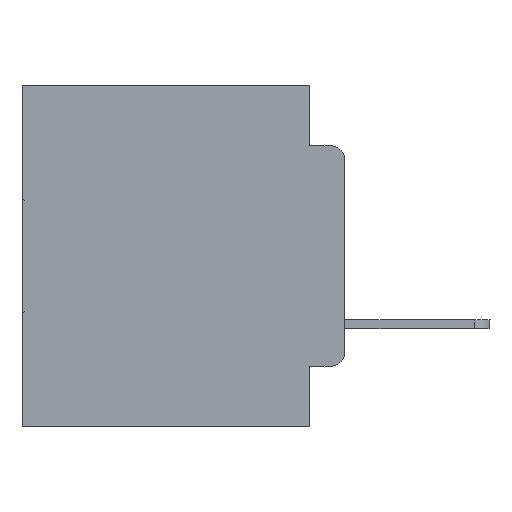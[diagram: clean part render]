
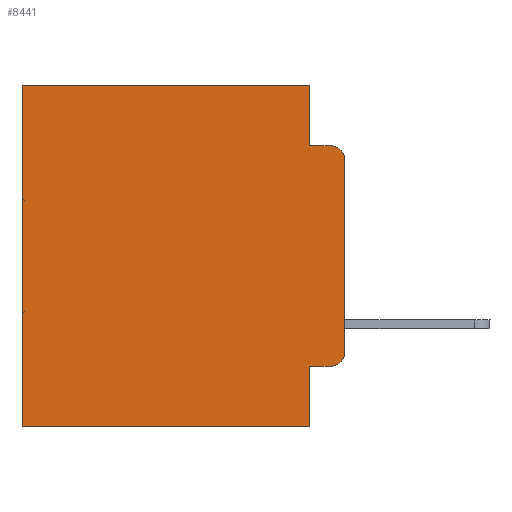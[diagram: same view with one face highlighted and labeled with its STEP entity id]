
A CAD part, left-side view. The second image highlights one B-rep face of the part: STEP entity #8441.
In plain terms, the highlighted planar face has unit normal (-1, 0, 0).
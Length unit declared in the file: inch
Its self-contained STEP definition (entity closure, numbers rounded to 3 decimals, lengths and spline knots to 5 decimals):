
#83 = DIRECTION ( 'NONE',  ( 0., 0., -1. ) ) ;
#173 = VERTEX_POINT ( 'NONE', #23700 ) ;
#396 = EDGE_CURVE ( 'NONE', #19547, #23823, #25147, .T. ) ;
#588 = EDGE_LOOP ( 'NONE', ( #3178, #11510, #20989, #927, #28662, #27290, #29901, #21959, #3169, #2044 ) ) ;
#727 = VECTOR ( 'NONE', #8855, 39.37008 ) ;
#927 = ORIENTED_EDGE ( 'NONE', *, *, #28316, .F. ) ;
#1236 = DIRECTION ( 'NONE',  ( 1., 0., 0. ) ) ;
#1614 = CARTESIAN_POINT ( 'NONE',  ( 0.298, 0.473, -0.5 ) ) ;
#1920 = CARTESIAN_POINT ( 'NONE',  ( 0.298, 0.051, -0.0885 ) ) ;
#2044 = ORIENTED_EDGE ( 'NONE', *, *, #396, .T. ) ;
#2188 = CARTESIAN_POINT ( 'NONE',  ( 0.298, 0.051, 0. ) ) ;
#2474 = CARTESIAN_POINT ( 'NONE',  ( 0.298, 0.473, 0. ) ) ;
#2804 = DIRECTION ( 'NONE',  ( 0., 0., -1. ) ) ;
#3169 = ORIENTED_EDGE ( 'NONE', *, *, #11675, .T. ) ;
#3178 = ORIENTED_EDGE ( 'NONE', *, *, #8367, .F. ) ;
#3919 = LINE ( 'NONE', #23243, #4625 ) ;
#4054 = VERTEX_POINT ( 'NONE', #20038 ) ;
#4377 = CARTESIAN_POINT ( 'NONE',  ( 0.298, 0.051, -0.4115 ) ) ;
#4625 = VECTOR ( 'NONE', #15830, 39.37008 ) ;
#4672 = LINE ( 'NONE', #16582, #15466 ) ;
#4869 = EDGE_CURVE ( 'NONE', #14816, #173, #23444, .T. ) ;
#5251 = VECTOR ( 'NONE', #28047, 39.37008 ) ;
#5938 = DIRECTION ( 'NONE',  ( -1., 0., 0. ) ) ;
#7000 = CARTESIAN_POINT ( 'NONE',  ( 0.298, 0.473, 0. ) ) ;
#7826 = VERTEX_POINT ( 'NONE', #1614 ) ;
#7828 = VERTEX_POINT ( 'NONE', #1920 ) ;
#8042 = VERTEX_POINT ( 'NONE', #24629 ) ;
#8151 = EDGE_CURVE ( 'NONE', #8042, #12135, #10025, .T. ) ;
#8367 = EDGE_CURVE ( 'NONE', #8042, #23823, #4672, .T. ) ;
#8441 = ADVANCED_FACE ( 'NONE', ( #19645 ), #12544, .F. ) ;
#8460 = LINE ( 'NONE', #27158, #19194 ) ;
#8855 = DIRECTION ( 'NONE',  ( 0., 0., -1. ) ) ;
#10025 = CIRCLE ( 'NONE', #13945, 0.02 ) ;
#10169 = DIRECTION ( 'NONE',  ( 0., -1., 0. ) ) ;
#10468 = VERTEX_POINT ( 'NONE', #7000 ) ;
#10725 = CARTESIAN_POINT ( 'NONE',  ( 0.298, 0.02, -0.1085 ) ) ;
#10935 = CARTESIAN_POINT ( 'NONE',  ( 0.298, 0.02, -0.4115 ) ) ;
#11510 = ORIENTED_EDGE ( 'NONE', *, *, #8151, .T. ) ;
#11675 = EDGE_CURVE ( 'NONE', #14816, #19547, #16623, .T. ) ;
#12135 = VERTEX_POINT ( 'NONE', #28130 ) ;
#12544 = PLANE ( 'NONE',  #14477 ) ;
#12732 = EDGE_CURVE ( 'NONE', #7828, #12135, #26395, .T. ) ;
#13470 = DIRECTION ( 'NONE',  ( 0., 0., -1. ) ) ;
#13795 = LINE ( 'NONE', #2188, #727 ) ;
#13945 = AXIS2_PLACEMENT_3D ( 'NONE', #10725, #5938, #24307 ) ;
#14163 = CARTESIAN_POINT ( 'NONE',  ( 0.298, 0.051, 0. ) ) ;
#14477 = AXIS2_PLACEMENT_3D ( 'NONE', #24586, #1236, #29521 ) ;
#14775 = AXIS2_PLACEMENT_3D ( 'NONE', #22905, #15789, #13470 ) ;
#14816 = VERTEX_POINT ( 'NONE', #4377 ) ;
#15466 = VECTOR ( 'NONE', #2804, 39.37008 ) ;
#15789 = DIRECTION ( 'NONE',  ( -1., 0., 0. ) ) ;
#15830 = DIRECTION ( 'NONE',  ( 0., 1., 0. ) ) ;
#15854 = EDGE_CURVE ( 'NONE', #4054, #10468, #8460, .T. ) ;
#16038 = VECTOR ( 'NONE', #83, 39.37008 ) ;
#16582 = CARTESIAN_POINT ( 'NONE',  ( 0.298, 0., 0. ) ) ;
#16623 = LINE ( 'NONE', #18322, #5251 ) ;
#16975 = CARTESIAN_POINT ( 'NONE',  ( 0.298, 0., -0.3915 ) ) ;
#18322 = CARTESIAN_POINT ( 'NONE',  ( 0.298, 0.051, -0.4115 ) ) ;
#19194 = VECTOR ( 'NONE', #29467, 39.37008 ) ;
#19547 = VERTEX_POINT ( 'NONE', #10935 ) ;
#19645 = FACE_OUTER_BOUND ( 'NONE', #588, .T. ) ;
#20038 = CARTESIAN_POINT ( 'NONE',  ( 0.298, 0.051, 0. ) ) ;
#20989 = ORIENTED_EDGE ( 'NONE', *, *, #12732, .F. ) ;
#21908 = CARTESIAN_POINT ( 'NONE',  ( 0.298, 0.051, -0.0885 ) ) ;
#21959 = ORIENTED_EDGE ( 'NONE', *, *, #4869, .F. ) ;
#22333 = VECTOR ( 'NONE', #30321, 39.37008 ) ;
#22905 = CARTESIAN_POINT ( 'NONE',  ( 0.298, 0.02, -0.3915 ) ) ;
#23243 = CARTESIAN_POINT ( 'NONE',  ( 0.298, 0., -0.5 ) ) ;
#23444 = LINE ( 'NONE', #14163, #16038 ) ;
#23700 = CARTESIAN_POINT ( 'NONE',  ( 0.298, 0.051, -0.5 ) ) ;
#23812 = LINE ( 'NONE', #2474, #22333 ) ;
#23823 = VERTEX_POINT ( 'NONE', #16975 ) ;
#24307 = DIRECTION ( 'NONE',  ( 0., 0., -1. ) ) ;
#24586 = CARTESIAN_POINT ( 'NONE',  ( 0.298, 0., 0. ) ) ;
#24629 = CARTESIAN_POINT ( 'NONE',  ( 0.298, 0., -0.1085 ) ) ;
#25147 = CIRCLE ( 'NONE', #14775, 0.02 ) ;
#25488 = EDGE_CURVE ( 'NONE', #173, #7826, #3919, .T. ) ;
#26395 = LINE ( 'NONE', #21908, #27507 ) ;
#27158 = CARTESIAN_POINT ( 'NONE',  ( 0.298, 0., 0. ) ) ;
#27290 = ORIENTED_EDGE ( 'NONE', *, *, #29564, .T. ) ;
#27507 = VECTOR ( 'NONE', #10169, 39.37008 ) ;
#28047 = DIRECTION ( 'NONE',  ( 0., -1., 0. ) ) ;
#28130 = CARTESIAN_POINT ( 'NONE',  ( 0.298, 0.02, -0.0885 ) ) ;
#28316 = EDGE_CURVE ( 'NONE', #4054, #7828, #13795, .T. ) ;
#28662 = ORIENTED_EDGE ( 'NONE', *, *, #15854, .T. ) ;
#29467 = DIRECTION ( 'NONE',  ( 0., 1., 0. ) ) ;
#29521 = DIRECTION ( 'NONE',  ( 0., 0., -1. ) ) ;
#29564 = EDGE_CURVE ( 'NONE', #10468, #7826, #23812, .T. ) ;
#29901 = ORIENTED_EDGE ( 'NONE', *, *, #25488, .F. ) ;
#30321 = DIRECTION ( 'NONE',  ( 0., 0., -1. ) ) ;
